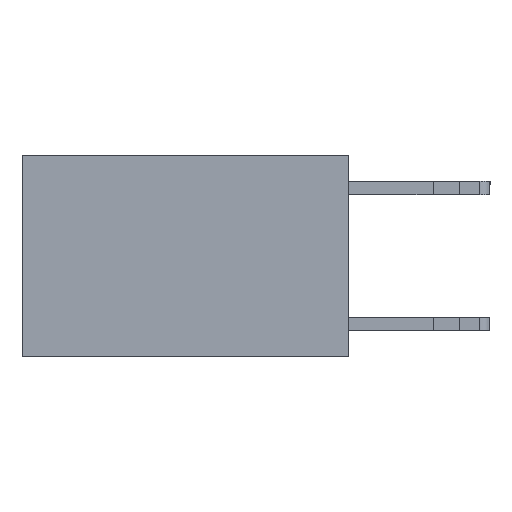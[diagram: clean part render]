
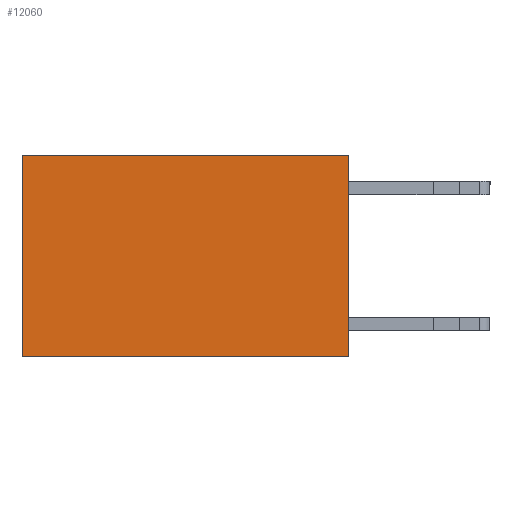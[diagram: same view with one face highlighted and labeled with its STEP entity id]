
A CAD part, left-side view. The second image highlights one B-rep face of the part: STEP entity #12060.
In plain terms, the highlighted planar face has unit normal (-1, 0, 0).
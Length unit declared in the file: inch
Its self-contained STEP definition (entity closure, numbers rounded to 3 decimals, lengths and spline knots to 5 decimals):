
#1818 = PLANE ( 'NONE',  #23889 ) ;
#2063 = LINE ( 'NONE', #13465, #10202 ) ;
#4053 = LINE ( 'NONE', #9753, #23411 ) ;
#4110 = VECTOR ( 'NONE', #12256, 39.37008 ) ;
#4226 = DIRECTION ( 'NONE',  ( 0., 1., 0. ) ) ;
#6275 = CARTESIAN_POINT ( 'NONE',  ( 0.2625, 0., 0. ) ) ;
#6661 = CARTESIAN_POINT ( 'NONE',  ( 0.2625, 0.6, 0. ) ) ;
#6937 = EDGE_CURVE ( 'NONE', #16513, #18464, #2063, .T. ) ;
#7101 = ORIENTED_EDGE ( 'NONE', *, *, #8963, .F. ) ;
#7166 = CARTESIAN_POINT ( 'NONE',  ( 0.2625, 0., 0. ) ) ;
#7288 = DIRECTION ( 'NONE',  ( 0., 0., -1. ) ) ;
#8963 = EDGE_CURVE ( 'NONE', #9891, #16513, #4053, .T. ) ;
#9284 = EDGE_CURVE ( 'NONE', #9891, #20877, #12900, .T. ) ;
#9359 = CARTESIAN_POINT ( 'NONE',  ( 0.2625, 0.6, -0.37 ) ) ;
#9753 = CARTESIAN_POINT ( 'NONE',  ( 0.2625, 0., 0. ) ) ;
#9891 = VERTEX_POINT ( 'NONE', #6275 ) ;
#10143 = CARTESIAN_POINT ( 'NONE',  ( 0.2625, 0.6, 0. ) ) ;
#10202 = VECTOR ( 'NONE', #4226, 39.37008 ) ;
#10590 = EDGE_LOOP ( 'NONE', ( #14123, #13948, #7101, #13217 ) ) ;
#12060 = ADVANCED_FACE ( 'NONE', ( #23903 ), #1818, .F. ) ;
#12256 = DIRECTION ( 'NONE',  ( 0., 0., -1. ) ) ;
#12427 = CARTESIAN_POINT ( 'NONE',  ( 0.2625, 0., 0. ) ) ;
#12900 = LINE ( 'NONE', #12427, #22648 ) ;
#13217 = ORIENTED_EDGE ( 'NONE', *, *, #9284, .T. ) ;
#13465 = CARTESIAN_POINT ( 'NONE',  ( 0.2625, 0., -0.37 ) ) ;
#13948 = ORIENTED_EDGE ( 'NONE', *, *, #6937, .F. ) ;
#14123 = ORIENTED_EDGE ( 'NONE', *, *, #20462, .T. ) ;
#15350 = DIRECTION ( 'NONE',  ( 0., 0., -1. ) ) ;
#16513 = VERTEX_POINT ( 'NONE', #23961 ) ;
#18346 = DIRECTION ( 'NONE',  ( 1., 0., 0. ) ) ;
#18464 = VERTEX_POINT ( 'NONE', #9359 ) ;
#19825 = DIRECTION ( 'NONE',  ( 0., 1., 0. ) ) ;
#20462 = EDGE_CURVE ( 'NONE', #20877, #18464, #23408, .T. ) ;
#20877 = VERTEX_POINT ( 'NONE', #10143 ) ;
#22648 = VECTOR ( 'NONE', #19825, 39.37008 ) ;
#23408 = LINE ( 'NONE', #6661, #4110 ) ;
#23411 = VECTOR ( 'NONE', #15350, 39.37008 ) ;
#23889 = AXIS2_PLACEMENT_3D ( 'NONE', #7166, #18346, #7288 ) ;
#23903 = FACE_OUTER_BOUND ( 'NONE', #10590, .T. ) ;
#23961 = CARTESIAN_POINT ( 'NONE',  ( 0.2625, 0., -0.37 ) ) ;
